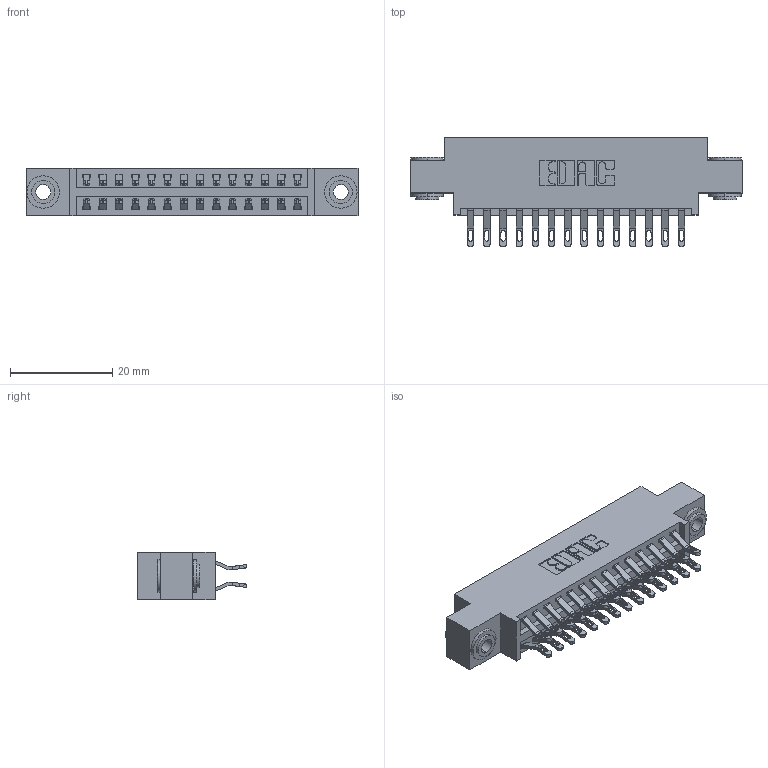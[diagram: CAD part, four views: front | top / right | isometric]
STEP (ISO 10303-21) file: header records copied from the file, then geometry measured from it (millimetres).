
FILE_DESCRIPTION (( 'STEP AP203' ), '1' );
FILE_NAME ('346-028-555-803.STEP', '2022-05-19T04:57:25', ( '' ), ( '' ), 'SwSTEP 2.0', 'SolidWorks 2020', '' );
FILE_SCHEMA (( 'CONFIG_CONTROL_DESIGN' ));
Length unit declared in the file: inch
Products named in the file (4): 345-292-001_555 Tail; 346 Part_0.170 Offset - 0.156 Dia-TH; 346-028-555-803; 345-250-002_345-250-002-102
Assembly tree (31 placements, depth 2):
  346-028-555-803
    346 Part_0.170 Offset - 0.156 Dia-TH
    345-292-001_555 Tail  x28
    345-250-002_345-250-002-102  x2
Bounding box: 65.02 x 21.46 x 9.4 mm (x, y, z)
Volume: 6051.1 mm3; surface area: 8595.4 mm2
Topology: 31 solids, 31 shells, 1802 faces, 5577 edges, 3714 vertices
Faces by surface type: plane 1028, cylinder 766, cone 8
Entity records: 14430 total; most frequent: CARTESIAN_POINT 2435, ORIENTED_EDGE 2330, DIRECTION 2195, EDGE_CURVE 1165, LINE 933, VECTOR 933, VERTEX_POINT 774, AXIS2_PLACEMENT_3D 631
